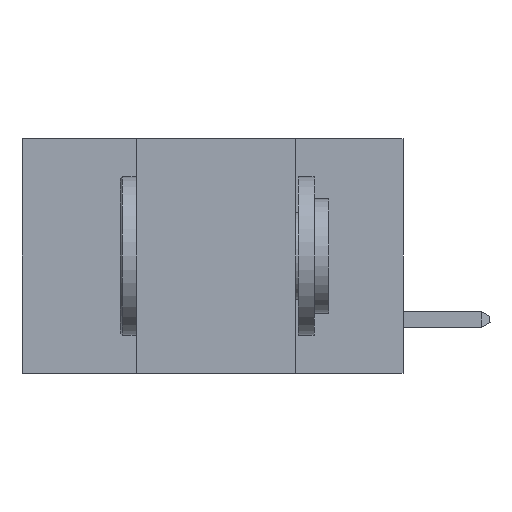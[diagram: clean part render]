
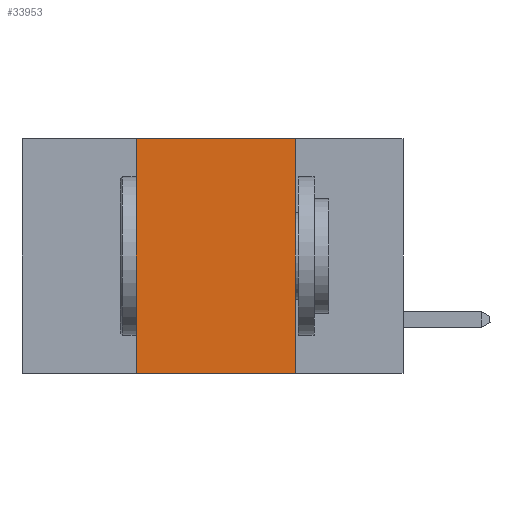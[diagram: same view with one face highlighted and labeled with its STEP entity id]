
A CAD part, left-side view. The second image highlights one B-rep face of the part: STEP entity #33953.
In plain terms, the highlighted planar face has unit normal (-1, 0, 0).
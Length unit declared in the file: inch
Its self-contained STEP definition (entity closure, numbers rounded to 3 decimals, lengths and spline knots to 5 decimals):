
#175 = VERTEX_POINT ( 'NONE', #43792 ) ;
#526 = CARTESIAN_POINT ( 'NONE',  ( 0., 0.17, 0. ) ) ;
#8328 = VERTEX_POINT ( 'NONE', #49100 ) ;
#9069 = VECTOR ( 'NONE', #29159, 39.37008 ) ;
#9637 = VERTEX_POINT ( 'NONE', #34855 ) ;
#10611 = EDGE_CURVE ( 'NONE', #8328, #9637, #36581, .T. ) ;
#15086 = LINE ( 'NONE', #32843, #9069 ) ;
#17013 = PLANE ( 'NONE',  #20604 ) ;
#17675 = LINE ( 'NONE', #32677, #49580 ) ;
#19131 = VERTEX_POINT ( 'NONE', #526 ) ;
#19400 = ORIENTED_EDGE ( 'NONE', *, *, #36180, .F. ) ;
#20604 = AXIS2_PLACEMENT_3D ( 'NONE', #44402, #21309, #20810 ) ;
#20810 = DIRECTION ( 'NONE',  ( 0., 0., -1. ) ) ;
#21309 = DIRECTION ( 'NONE',  ( 1., 0., 0. ) ) ;
#22160 = DIRECTION ( 'NONE',  ( 0., -1., 0. ) ) ;
#22332 = EDGE_LOOP ( 'NONE', ( #23910, #19400, #28865, #47813 ) ) ;
#23910 = ORIENTED_EDGE ( 'NONE', *, *, #24906, .F. ) ;
#24906 = EDGE_CURVE ( 'NONE', #19131, #9637, #24935, .T. ) ;
#24935 = LINE ( 'NONE', #27069, #32126 ) ;
#26366 = VECTOR ( 'NONE', #22160, 39.37008 ) ;
#27069 = CARTESIAN_POINT ( 'NONE',  ( 0., 0.17, 0. ) ) ;
#27622 = EDGE_CURVE ( 'NONE', #8328, #175, #15086, .T. ) ;
#28865 = ORIENTED_EDGE ( 'NONE', *, *, #27622, .F. ) ;
#29159 = DIRECTION ( 'NONE',  ( 0., 0., 1. ) ) ;
#30312 = FACE_OUTER_BOUND ( 'NONE', #22332, .T. ) ;
#32126 = VECTOR ( 'NONE', #46273, 39.37008 ) ;
#32677 = CARTESIAN_POINT ( 'NONE',  ( 0., 0.6, 0. ) ) ;
#32843 = CARTESIAN_POINT ( 'NONE',  ( 0., 0.42, 0. ) ) ;
#33953 = ADVANCED_FACE ( 'NONE', ( #30312 ), #17013, .F. ) ;
#34855 = CARTESIAN_POINT ( 'NONE',  ( 0., 0.17, -0.37 ) ) ;
#36180 = EDGE_CURVE ( 'NONE', #175, #19131, #17675, .T. ) ;
#36581 = LINE ( 'NONE', #44765, #26366 ) ;
#40265 = DIRECTION ( 'NONE',  ( 0., -1., 0. ) ) ;
#43792 = CARTESIAN_POINT ( 'NONE',  ( 0., 0.42, 0. ) ) ;
#44402 = CARTESIAN_POINT ( 'NONE',  ( 0., 0.6, 0. ) ) ;
#44765 = CARTESIAN_POINT ( 'NONE',  ( 0., 0.6, -0.37 ) ) ;
#46273 = DIRECTION ( 'NONE',  ( 0., 0., -1. ) ) ;
#47813 = ORIENTED_EDGE ( 'NONE', *, *, #10611, .T. ) ;
#49100 = CARTESIAN_POINT ( 'NONE',  ( 0., 0.42, -0.37 ) ) ;
#49580 = VECTOR ( 'NONE', #40265, 39.37008 ) ;
